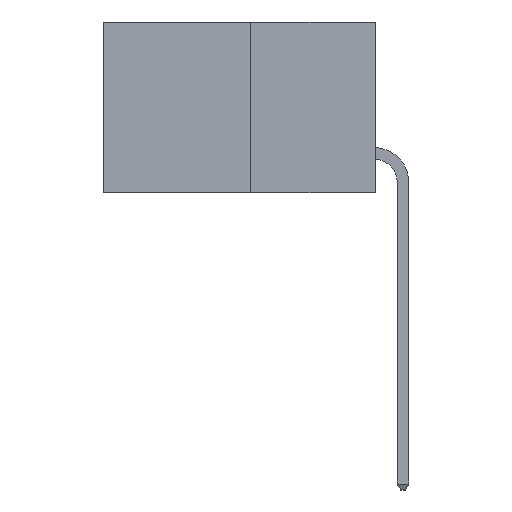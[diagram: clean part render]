
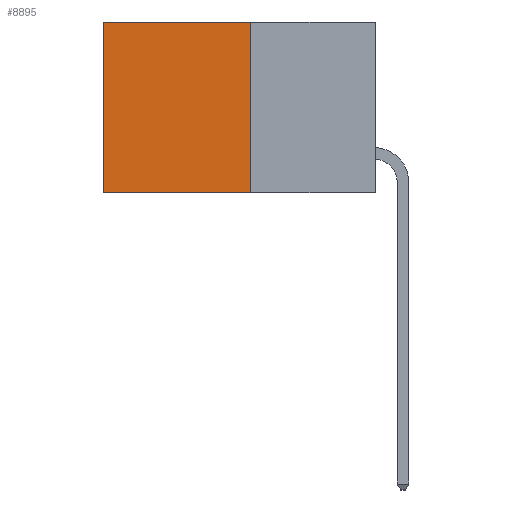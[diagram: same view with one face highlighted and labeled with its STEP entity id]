
A CAD part, left-side view. The second image highlights one B-rep face of the part: STEP entity #8895.
In plain terms, the highlighted planar face has unit normal (-1, 0, 0).
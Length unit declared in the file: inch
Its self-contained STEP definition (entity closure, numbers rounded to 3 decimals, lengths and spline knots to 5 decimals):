
#131 = VERTEX_POINT ( 'NONE', #1814 ) ;
#602 = LINE ( 'NONE', #5779, #7002 ) ;
#999 = DIRECTION ( 'NONE',  ( 1., 0., 0. ) ) ;
#1201 = ORIENTED_EDGE ( 'NONE', *, *, #10330, .F. ) ;
#1252 = LINE ( 'NONE', #7207, #3345 ) ;
#1532 = EDGE_CURVE ( 'NONE', #131, #4502, #5277, .T. ) ;
#1706 = VERTEX_POINT ( 'NONE', #5622 ) ;
#1814 = CARTESIAN_POINT ( 'NONE',  ( 0.277, 0.27, 0. ) ) ;
#2742 = CARTESIAN_POINT ( 'NONE',  ( 0.277, 0.59, -0.37 ) ) ;
#2832 = DIRECTION ( 'NONE',  ( 0., 0., -1. ) ) ;
#3261 = EDGE_CURVE ( 'NONE', #131, #1706, #1252, .T. ) ;
#3345 = VECTOR ( 'NONE', #7469, 39.37008 ) ;
#3374 = EDGE_CURVE ( 'NONE', #1706, #5272, #8998, .T. ) ;
#4502 = VERTEX_POINT ( 'NONE', #6096 ) ;
#4630 = CARTESIAN_POINT ( 'NONE',  ( 0.277, 0.59, -0.37 ) ) ;
#5025 = VECTOR ( 'NONE', #7021, 39.37008 ) ;
#5272 = VERTEX_POINT ( 'NONE', #4630 ) ;
#5277 = LINE ( 'NONE', #7425, #5025 ) ;
#5554 = AXIS2_PLACEMENT_3D ( 'NONE', #5771, #999, #6594 ) ;
#5622 = CARTESIAN_POINT ( 'NONE',  ( 0.277, 0.59, 0. ) ) ;
#5771 = CARTESIAN_POINT ( 'NONE',  ( 0.277, 0.27, -0.37 ) ) ;
#5779 = CARTESIAN_POINT ( 'NONE',  ( 0.277, 0.27, -0.37 ) ) ;
#5809 = ORIENTED_EDGE ( 'NONE', *, *, #3261, .T. ) ;
#6096 = CARTESIAN_POINT ( 'NONE',  ( 0.277, 0.27, -0.37 ) ) ;
#6594 = DIRECTION ( 'NONE',  ( 0., 0., -1. ) ) ;
#6752 = DIRECTION ( 'NONE',  ( 0., 1., 0. ) ) ;
#7002 = VECTOR ( 'NONE', #6752, 39.37008 ) ;
#7021 = DIRECTION ( 'NONE',  ( 0., 0., -1. ) ) ;
#7207 = CARTESIAN_POINT ( 'NONE',  ( 0.277, 0.27, 0. ) ) ;
#7425 = CARTESIAN_POINT ( 'NONE',  ( 0.277, 0.27, -0.37 ) ) ;
#7469 = DIRECTION ( 'NONE',  ( 0., 1., 0. ) ) ;
#7939 = ORIENTED_EDGE ( 'NONE', *, *, #3374, .T. ) ;
#8048 = EDGE_LOOP ( 'NONE', ( #7939, #1201, #9325, #5809 ) ) ;
#8492 = VECTOR ( 'NONE', #2832, 39.37008 ) ;
#8895 = ADVANCED_FACE ( 'NONE', ( #9198 ), #9784, .F. ) ;
#8998 = LINE ( 'NONE', #2742, #8492 ) ;
#9198 = FACE_OUTER_BOUND ( 'NONE', #8048, .T. ) ;
#9325 = ORIENTED_EDGE ( 'NONE', *, *, #1532, .F. ) ;
#9784 = PLANE ( 'NONE',  #5554 ) ;
#10330 = EDGE_CURVE ( 'NONE', #4502, #5272, #602, .T. ) ;
